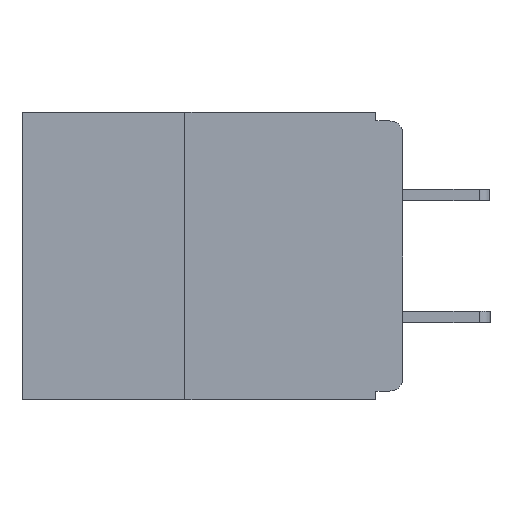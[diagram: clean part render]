
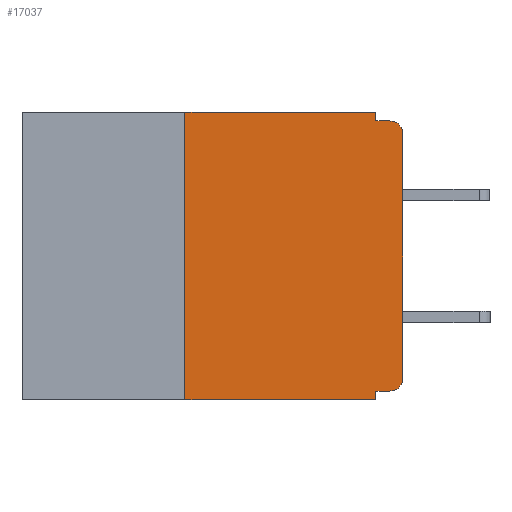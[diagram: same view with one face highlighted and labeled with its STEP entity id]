
A CAD part, left-side view. The second image highlights one B-rep face of the part: STEP entity #17037.
In plain terms, the highlighted planar face has unit normal (-1, 0, 0).
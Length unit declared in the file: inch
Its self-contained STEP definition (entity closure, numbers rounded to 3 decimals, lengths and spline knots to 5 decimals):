
#276 = CARTESIAN_POINT ( 'NONE',  ( 0., 0., 0. ) ) ;
#891 = VECTOR ( 'NONE', #18619, 39.37008 ) ;
#1057 = CARTESIAN_POINT ( 'NONE',  ( 0., 0.015, -0.32 ) ) ;
#1148 = EDGE_CURVE ( 'NONE', #19496, #26970, #14767, .T. ) ;
#1281 = VECTOR ( 'NONE', #22494, 39.37008 ) ;
#1488 = EDGE_CURVE ( 'NONE', #8107, #20590, #13694, .T. ) ;
#1606 = LINE ( 'NONE', #16391, #891 ) ;
#1741 = PLANE ( 'NONE',  #19714 ) ;
#1840 = DIRECTION ( 'NONE',  ( 0., 0., -1. ) ) ;
#1992 = EDGE_CURVE ( 'NONE', #8107, #16405, #23312, .T. ) ;
#2636 = EDGE_CURVE ( 'NONE', #20590, #17678, #13982, .T. ) ;
#3150 = CARTESIAN_POINT ( 'NONE',  ( 0., 0.031, -0.32 ) ) ;
#4784 = LINE ( 'NONE', #7093, #15974 ) ;
#5222 = DIRECTION ( 'NONE',  ( 0., 0., -1. ) ) ;
#5344 = DIRECTION ( 'NONE',  ( 0., 0., 1. ) ) ;
#5376 = CARTESIAN_POINT ( 'NONE',  ( 0., 0.031, -0.01 ) ) ;
#7062 = DIRECTION ( 'NONE',  ( 0., 0., -1. ) ) ;
#7093 = CARTESIAN_POINT ( 'NONE',  ( 0., 0.031, 0. ) ) ;
#7099 = CARTESIAN_POINT ( 'NONE',  ( 0., 0.25, 0. ) ) ;
#7256 = CARTESIAN_POINT ( 'NONE',  ( 0., 0.015, -0.305 ) ) ;
#7389 = CARTESIAN_POINT ( 'NONE',  ( 0., 0., -0.32 ) ) ;
#7801 = EDGE_CURVE ( 'NONE', #17690, #10313, #4784, .T. ) ;
#7865 = CARTESIAN_POINT ( 'NONE',  ( 0., 0.031, -0.33 ) ) ;
#8107 = VERTEX_POINT ( 'NONE', #1057 ) ;
#8157 = DIRECTION ( 'NONE',  ( 0., 0., -1. ) ) ;
#8187 = DIRECTION ( 'NONE',  ( -1., 0., 0. ) ) ;
#8494 = CARTESIAN_POINT ( 'NONE',  ( 0., 0., -0.025 ) ) ;
#8776 = EDGE_CURVE ( 'NONE', #10313, #26970, #9268, .T. ) ;
#8808 = FACE_OUTER_BOUND ( 'NONE', #23045, .T. ) ;
#9268 = LINE ( 'NONE', #24483, #14565 ) ;
#9692 = CARTESIAN_POINT ( 'NONE',  ( 0., 0.25, -0.33 ) ) ;
#10200 = EDGE_CURVE ( 'NONE', #16405, #19496, #20047, .T. ) ;
#10313 = VERTEX_POINT ( 'NONE', #5376 ) ;
#10722 = VERTEX_POINT ( 'NONE', #7099 ) ;
#10822 = CARTESIAN_POINT ( 'NONE',  ( 0., 0.437, 0. ) ) ;
#11264 = DIRECTION ( 'NONE',  ( 0., -1., 0. ) ) ;
#11737 = DIRECTION ( 'NONE',  ( 0., 1., 0. ) ) ;
#12134 = CARTESIAN_POINT ( 'NONE',  ( 0., 0.25, -0.33 ) ) ;
#12184 = ORIENTED_EDGE ( 'NONE', *, *, #1992, .T. ) ;
#12951 = ORIENTED_EDGE ( 'NONE', *, *, #1488, .F. ) ;
#13000 = VECTOR ( 'NONE', #11737, 39.37008 ) ;
#13085 = LINE ( 'NONE', #12134, #24115 ) ;
#13258 = CARTESIAN_POINT ( 'NONE',  ( 0., 0., -0.305 ) ) ;
#13302 = ORIENTED_EDGE ( 'NONE', *, *, #2636, .F. ) ;
#13694 = LINE ( 'NONE', #7389, #13000 ) ;
#13982 = LINE ( 'NONE', #7865, #1281 ) ;
#14096 = EDGE_CURVE ( 'NONE', #23934, #17678, #1606, .T. ) ;
#14565 = VECTOR ( 'NONE', #11264, 39.37008 ) ;
#14766 = ORIENTED_EDGE ( 'NONE', *, *, #22366, .F. ) ;
#14767 = CIRCLE ( 'NONE', #23800, 0.015 ) ;
#15294 = DIRECTION ( 'NONE',  ( 1., 0., 0. ) ) ;
#15974 = VECTOR ( 'NONE', #7062, 39.37008 ) ;
#16391 = CARTESIAN_POINT ( 'NONE',  ( 0., 0.437, -0.33 ) ) ;
#16405 = VERTEX_POINT ( 'NONE', #13258 ) ;
#17037 = ADVANCED_FACE ( 'NONE', ( #8808 ), #1741, .F. ) ;
#17181 = LINE ( 'NONE', #23558, #27983 ) ;
#17410 = ORIENTED_EDGE ( 'NONE', *, *, #1148, .T. ) ;
#17678 = VERTEX_POINT ( 'NONE', #28227 ) ;
#17690 = VERTEX_POINT ( 'NONE', #26184 ) ;
#18619 = DIRECTION ( 'NONE',  ( 0., -1., 0. ) ) ;
#19187 = ORIENTED_EDGE ( 'NONE', *, *, #10200, .T. ) ;
#19375 = VECTOR ( 'NONE', #26894, 39.37008 ) ;
#19496 = VERTEX_POINT ( 'NONE', #8494 ) ;
#19714 = AXIS2_PLACEMENT_3D ( 'NONE', #10822, #15294, #1840 ) ;
#19775 = ORIENTED_EDGE ( 'NONE', *, *, #8776, .F. ) ;
#20047 = LINE ( 'NONE', #276, #19375 ) ;
#20590 = VERTEX_POINT ( 'NONE', #3150 ) ;
#20890 = ORIENTED_EDGE ( 'NONE', *, *, #7801, .F. ) ;
#21936 = ORIENTED_EDGE ( 'NONE', *, *, #14096, .T. ) ;
#22366 = EDGE_CURVE ( 'NONE', #23934, #10722, #13085, .T. ) ;
#22494 = DIRECTION ( 'NONE',  ( 0., 0., -1. ) ) ;
#23045 = EDGE_LOOP ( 'NONE', ( #19187, #17410, #19775, #20890, #24290, #14766, #21936, #13302, #12951, #12184 ) ) ;
#23312 = CIRCLE ( 'NONE', #25099, 0.015 ) ;
#23494 = CARTESIAN_POINT ( 'NONE',  ( 0., 0.015, -0.01 ) ) ;
#23558 = CARTESIAN_POINT ( 'NONE',  ( 0., 0.437, 0. ) ) ;
#23800 = AXIS2_PLACEMENT_3D ( 'NONE', #27549, #27526, #5222 ) ;
#23934 = VERTEX_POINT ( 'NONE', #9692 ) ;
#24115 = VECTOR ( 'NONE', #5344, 39.37008 ) ;
#24290 = ORIENTED_EDGE ( 'NONE', *, *, #27598, .F. ) ;
#24483 = CARTESIAN_POINT ( 'NONE',  ( 0., 0., -0.01 ) ) ;
#25099 = AXIS2_PLACEMENT_3D ( 'NONE', #7256, #8187, #8157 ) ;
#25749 = DIRECTION ( 'NONE',  ( 0., -1., 0. ) ) ;
#26184 = CARTESIAN_POINT ( 'NONE',  ( 0., 0.031, 0. ) ) ;
#26894 = DIRECTION ( 'NONE',  ( 0., 0., 1. ) ) ;
#26970 = VERTEX_POINT ( 'NONE', #23494 ) ;
#27526 = DIRECTION ( 'NONE',  ( -1., 0., 0. ) ) ;
#27549 = CARTESIAN_POINT ( 'NONE',  ( 0., 0.015, -0.025 ) ) ;
#27598 = EDGE_CURVE ( 'NONE', #10722, #17690, #17181, .T. ) ;
#27983 = VECTOR ( 'NONE', #25749, 39.37008 ) ;
#28227 = CARTESIAN_POINT ( 'NONE',  ( 0., 0.031, -0.33 ) ) ;
